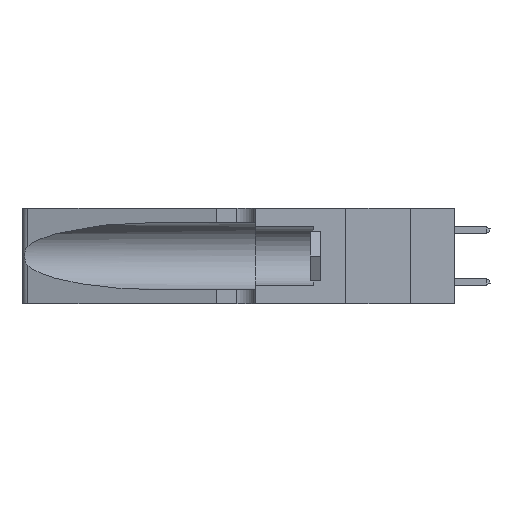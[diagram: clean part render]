
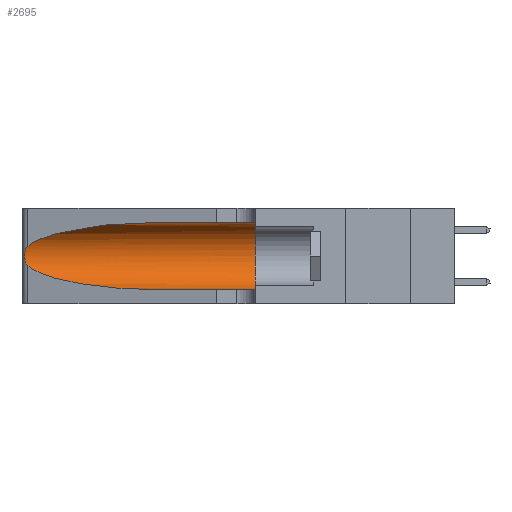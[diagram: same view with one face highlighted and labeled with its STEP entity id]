
A CAD part, left-side view. The second image highlights one B-rep face of the part: STEP entity #2695.
In plain terms, the highlighted cylindrical face has radius 3.308 mm (diameter 6.617 mm), a partial arc.
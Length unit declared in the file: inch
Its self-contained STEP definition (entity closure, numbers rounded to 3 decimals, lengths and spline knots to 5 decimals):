
#278 = CARTESIAN_POINT ( 'NONE',  ( 0.26018, 1.23835, 0.19895 ) ) ;
#366 = CARTESIAN_POINT ( 'NONE',  ( 0.25856, 1.23593, 0.16098 ) ) ;
#623 = LINE ( 'NONE', #18359, #3205 ) ;
#1664 = B_SPLINE_CURVE_WITH_KNOTS ( 'NONE', 3,
 ( #13292, #22171, #22097, #20355, #11204, #278, #18534, #14935, #5953, #366, #22330, #4045, #5780, #13047 ),
 .UNSPECIFIED., .F., .F.,
 ( 4, 2, 2, 2, 2, 2, 4 ),
 ( 0., 0.00027, 0.00053, 0.00107, 0.0016, 0.00187, 0.00214 ),
 .UNSPECIFIED. ) ;
#2226 = ORIENTED_EDGE ( 'NONE', *, *, #21895, .T. ) ;
#2386 = AXIS2_PLACEMENT_3D ( 'NONE', #12642, #3720, #18292 ) ;
#2575 = CARTESIAN_POINT ( 'NONE',  ( 0.1305, 0.35, 0.185 ) ) ;
#2695 = ADVANCED_FACE ( 'NONE', ( #7359 ), #10219, .F. ) ;
#3205 = VECTOR ( 'NONE', #9291, 39.37008 ) ;
#3720 = DIRECTION ( 'NONE',  ( 0., -1., 0. ) ) ;
#3980 = CARTESIAN_POINT ( 'NONE',  ( 0.18966, 0.96281, 0.31525 ) ) ;
#4045 = CARTESIAN_POINT ( 'NONE',  ( 0.25639, 1.23186, 0.15144 ) ) ;
#4674 = VERTEX_POINT ( 'NONE', #19252 ) ;
#5780 = CARTESIAN_POINT ( 'NONE',  ( 0.25555, 1.22993, 0.14849 ) ) ;
#5953 = CARTESIAN_POINT ( 'NONE',  ( 0.26017, 1.23833, 0.17102 ) ) ;
#6303 = VERTEX_POINT ( 'NONE', #8745 ) ;
#6672 = EDGE_CURVE ( 'NONE', #23292, #6303, #7175, .T. ) ;
#6681 = CARTESIAN_POINT ( 'NONE',  ( 0.1305, 0.72297, 0.05475 ) ) ;
#6867 = EDGE_LOOP ( 'NONE', ( #19654, #2226, #12150, #20317, #17370, #18399 ) ) ;
#7175 = LINE ( 'NONE', #8905, #20535 ) ;
#7358 = CARTESIAN_POINT ( 'NONE',  ( 0.2373, 1.15595, 0.08982 ) ) ;
#7359 = FACE_OUTER_BOUND ( 'NONE', #6867, .T. ) ;
#7593 = CARTESIAN_POINT ( 'NONE',  ( 0.25487, 1.22718, 0.22369 ) ) ;
#8745 = CARTESIAN_POINT ( 'NONE',  ( 0.1305, 0.35, 0.31525 ) ) ;
#8905 = CARTESIAN_POINT ( 'NONE',  ( 0.1305, 1.61858, 0.31525 ) ) ;
#9056 = CIRCLE ( 'NONE', #14762, 0.13025 ) ;
#9262 = VERTEX_POINT ( 'NONE', #6681 ) ;
#9291 = DIRECTION ( 'NONE',  ( 0., -1., 0. ) ) ;
#10182 = CARTESIAN_POINT ( 'NONE',  ( 0.1305, 0.72297, 0.05475 ) ) ;
#10219 = CYLINDRICAL_SURFACE ( 'NONE', #2386, 0.13025 ) ;
#10586 =( BOUNDED_CURVE ( )  B_SPLINE_CURVE ( 3, ( #18465, #3980, #11148, #7593 ),
 .UNSPECIFIED., .F., .T. ) 
 B_SPLINE_CURVE_WITH_KNOTS ( ( 4, 4 ),
 ( 1.5708, 2.84003 ),
 .UNSPECIFIED. ) 
 CURVE ( )  GEOMETRIC_REPRESENTATION_ITEM ( )  RATIONAL_B_SPLINE_CURVE ( ( 1., 0.87, 0.87, 1. ) ) 
 REPRESENTATION_ITEM ( '' )  );
#11148 = CARTESIAN_POINT ( 'NONE',  ( 0.2373, 1.15595, 0.28018 ) ) ;
#11204 = CARTESIAN_POINT ( 'NONE',  ( 0.25854, 1.2359, 0.20912 ) ) ;
#11274 = CARTESIAN_POINT ( 'NONE',  ( 0.18966, 0.96281, 0.05475 ) ) ;
#12150 = ORIENTED_EDGE ( 'NONE', *, *, #17802, .T. ) ;
#12642 = CARTESIAN_POINT ( 'NONE',  ( 0.1305, 1.61858, 0.185 ) ) ;
#12914 =( BOUNDED_CURVE ( )  B_SPLINE_CURVE ( 3, ( #19920, #7358, #11274, #10182 ),
 .UNSPECIFIED., .F., .T. ) 
 B_SPLINE_CURVE_WITH_KNOTS ( ( 4, 4 ),
 ( 3.44316, 4.71239 ),
 .UNSPECIFIED. ) 
 CURVE ( )  GEOMETRIC_REPRESENTATION_ITEM ( )  RATIONAL_B_SPLINE_CURVE ( ( 1., 0.87, 0.87, 1. ) ) 
 REPRESENTATION_ITEM ( '' )  );
#13047 = CARTESIAN_POINT ( 'NONE',  ( 0.25487, 1.22718, 0.14631 ) ) ;
#13292 = CARTESIAN_POINT ( 'NONE',  ( 0.25487, 1.22718, 0.22369 ) ) ;
#14306 = EDGE_CURVE ( 'NONE', #6303, #4674, #9056, .T. ) ;
#14762 = AXIS2_PLACEMENT_3D ( 'NONE', #2575, #16995, #18834 ) ;
#14935 = CARTESIAN_POINT ( 'NONE',  ( 0.26075, 1.23896, 0.178 ) ) ;
#15506 = CARTESIAN_POINT ( 'NONE',  ( 0.1305, 0.72297, 0.31525 ) ) ;
#16995 = DIRECTION ( 'NONE',  ( 0., 1., 0. ) ) ;
#17370 = ORIENTED_EDGE ( 'NONE', *, *, #14306, .F. ) ;
#17802 = EDGE_CURVE ( 'NONE', #21510, #9262, #12914, .T. ) ;
#18059 = CARTESIAN_POINT ( 'NONE',  ( 0.25487, 1.22718, 0.14631 ) ) ;
#18292 = DIRECTION ( 'NONE',  ( 0., 0., -1. ) ) ;
#18359 = CARTESIAN_POINT ( 'NONE',  ( 0.1305, 1.61858, 0.05475 ) ) ;
#18399 = ORIENTED_EDGE ( 'NONE', *, *, #6672, .F. ) ;
#18465 = CARTESIAN_POINT ( 'NONE',  ( 0.1305, 0.72297, 0.31525 ) ) ;
#18534 = CARTESIAN_POINT ( 'NONE',  ( 0.26075, 1.23896, 0.19203 ) ) ;
#18834 = DIRECTION ( 'NONE',  ( 0., 0., 1. ) ) ;
#19252 = CARTESIAN_POINT ( 'NONE',  ( 0.1305, 0.35, 0.05475 ) ) ;
#19654 = ORIENTED_EDGE ( 'NONE', *, *, #23161, .T. ) ;
#19920 = CARTESIAN_POINT ( 'NONE',  ( 0.25487, 1.22718, 0.14631 ) ) ;
#20317 = ORIENTED_EDGE ( 'NONE', *, *, #23533, .T. ) ;
#20355 = CARTESIAN_POINT ( 'NONE',  ( 0.25787, 1.23484, 0.2124 ) ) ;
#20535 = VECTOR ( 'NONE', #23450, 39.37008 ) ;
#21510 = VERTEX_POINT ( 'NONE', #18059 ) ;
#21895 = EDGE_CURVE ( 'NONE', #22679, #21510, #1664, .T. ) ;
#22097 = CARTESIAN_POINT ( 'NONE',  ( 0.25639, 1.23184, 0.21858 ) ) ;
#22171 = CARTESIAN_POINT ( 'NONE',  ( 0.25555, 1.22994, 0.2215 ) ) ;
#22330 = CARTESIAN_POINT ( 'NONE',  ( 0.25789, 1.23486, 0.15765 ) ) ;
#22679 = VERTEX_POINT ( 'NONE', #22704 ) ;
#22704 = CARTESIAN_POINT ( 'NONE',  ( 0.25487, 1.22718, 0.22369 ) ) ;
#23161 = EDGE_CURVE ( 'NONE', #23292, #22679, #10586, .T. ) ;
#23292 = VERTEX_POINT ( 'NONE', #15506 ) ;
#23450 = DIRECTION ( 'NONE',  ( 0., -1., 0. ) ) ;
#23533 = EDGE_CURVE ( 'NONE', #9262, #4674, #623, .T. ) ;
